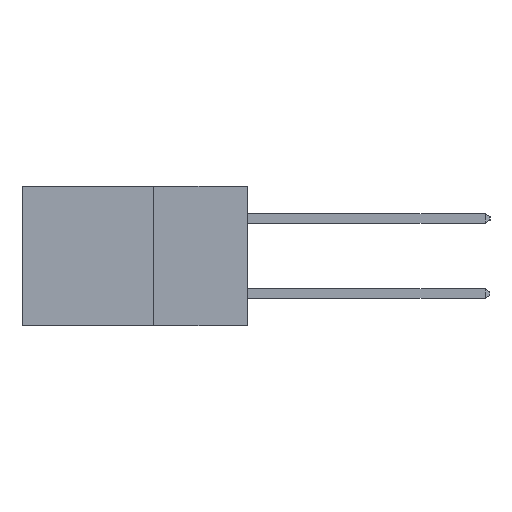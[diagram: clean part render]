
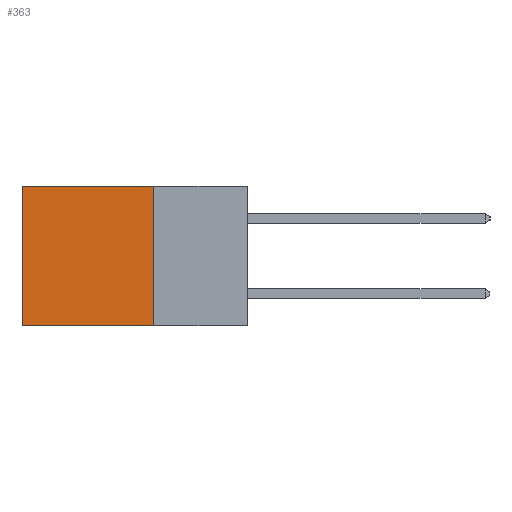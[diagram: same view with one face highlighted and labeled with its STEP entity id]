
A CAD part, left-side view. The second image highlights one B-rep face of the part: STEP entity #363.
In plain terms, the highlighted planar face has unit normal (-1, 0, 0).
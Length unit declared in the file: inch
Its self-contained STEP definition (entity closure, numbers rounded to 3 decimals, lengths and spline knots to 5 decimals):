
#363 = ADVANCED_FACE ( 'NONE', ( #2819 ), #3012, .F. ) ;
#451 = CARTESIAN_POINT ( 'NONE',  ( 0.298, 0.25, 0. ) ) ;
#1377 = DIRECTION ( 'NONE',  ( 0., 0., -1. ) ) ;
#1474 = ORIENTED_EDGE ( 'NONE', *, *, #6920, .F. ) ;
#1759 = LINE ( 'NONE', #11411, #4729 ) ;
#1913 = EDGE_LOOP ( 'NONE', ( #6708, #1474, #13988, #12328 ) ) ;
#2331 = VERTEX_POINT ( 'NONE', #6452 ) ;
#2819 = FACE_OUTER_BOUND ( 'NONE', #1913, .T. ) ;
#3012 = PLANE ( 'NONE',  #6471 ) ;
#3123 = CARTESIAN_POINT ( 'NONE',  ( 0.298, 0.25, 0. ) ) ;
#4722 = DIRECTION ( 'NONE',  ( 0., 1., 0. ) ) ;
#4729 = VECTOR ( 'NONE', #4722, 39.37008 ) ;
#4804 = CARTESIAN_POINT ( 'NONE',  ( 0.298, 0.25, -0.37 ) ) ;
#5216 = VERTEX_POINT ( 'NONE', #10845 ) ;
#5702 = DIRECTION ( 'NONE',  ( 0., 0., -1. ) ) ;
#6452 = CARTESIAN_POINT ( 'NONE',  ( 0.298, 0.6, 0. ) ) ;
#6471 = AXIS2_PLACEMENT_3D ( 'NONE', #3123, #10194, #1377 ) ;
#6708 = ORIENTED_EDGE ( 'NONE', *, *, #8264, .T. ) ;
#6920 = EDGE_CURVE ( 'NONE', #14456, #5216, #8068, .T. ) ;
#7307 = LINE ( 'NONE', #7965, #12514 ) ;
#7965 = CARTESIAN_POINT ( 'NONE',  ( 0.298, 0.6, 0. ) ) ;
#8068 = LINE ( 'NONE', #4804, #13681 ) ;
#8132 = DIRECTION ( 'NONE',  ( 0., 1., 0. ) ) ;
#8264 = EDGE_CURVE ( 'NONE', #2331, #5216, #7307, .T. ) ;
#8527 = VERTEX_POINT ( 'NONE', #14134 ) ;
#9471 = VECTOR ( 'NONE', #10523, 39.37008 ) ;
#9807 = LINE ( 'NONE', #451, #9471 ) ;
#10194 = DIRECTION ( 'NONE',  ( 1., 0., 0. ) ) ;
#10523 = DIRECTION ( 'NONE',  ( 0., 0., -1. ) ) ;
#10845 = CARTESIAN_POINT ( 'NONE',  ( 0.298, 0.6, -0.37 ) ) ;
#11167 = CARTESIAN_POINT ( 'NONE',  ( 0.298, 0.25, -0.37 ) ) ;
#11411 = CARTESIAN_POINT ( 'NONE',  ( 0.298, 0.25, 0. ) ) ;
#12328 = ORIENTED_EDGE ( 'NONE', *, *, #12619, .T. ) ;
#12514 = VECTOR ( 'NONE', #5702, 39.37008 ) ;
#12619 = EDGE_CURVE ( 'NONE', #8527, #2331, #1759, .T. ) ;
#13393 = EDGE_CURVE ( 'NONE', #8527, #14456, #9807, .T. ) ;
#13681 = VECTOR ( 'NONE', #8132, 39.37008 ) ;
#13988 = ORIENTED_EDGE ( 'NONE', *, *, #13393, .F. ) ;
#14134 = CARTESIAN_POINT ( 'NONE',  ( 0.298, 0.25, 0. ) ) ;
#14456 = VERTEX_POINT ( 'NONE', #11167 ) ;
